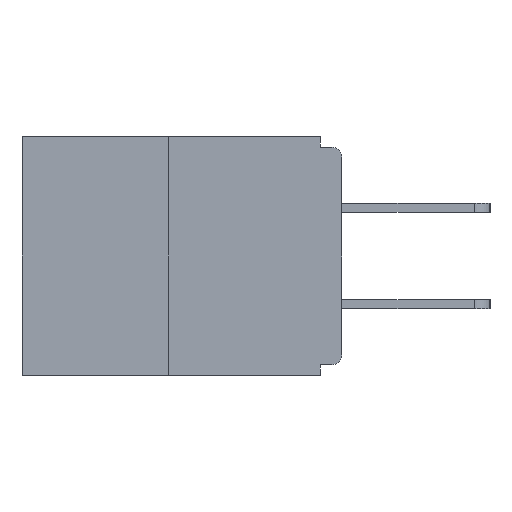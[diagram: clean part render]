
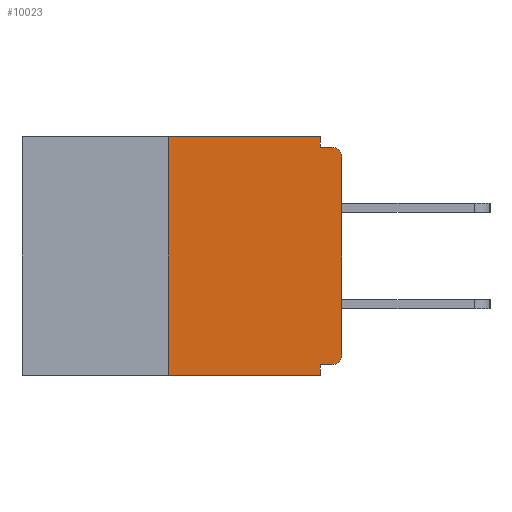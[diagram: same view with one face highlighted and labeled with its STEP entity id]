
A CAD part, left-side view. The second image highlights one B-rep face of the part: STEP entity #10023.
In plain terms, the highlighted planar face has unit normal (-1, 0, 0).
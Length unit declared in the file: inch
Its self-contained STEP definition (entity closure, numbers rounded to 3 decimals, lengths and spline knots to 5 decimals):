
#547 = CARTESIAN_POINT ( 'NONE',  ( 0., 0.25, 0. ) ) ;
#806 = EDGE_CURVE ( 'NONE', #11763, #2201, #15070, .T. ) ;
#1167 = DIRECTION ( 'NONE',  ( 0., -1., 0. ) ) ;
#1571 = VECTOR ( 'NONE', #18775, 39.37008 ) ;
#1791 = EDGE_CURVE ( 'NONE', #5650, #12004, #2619, .T. ) ;
#1837 = DIRECTION ( 'NONE',  ( 0., 0., 1. ) ) ;
#2201 = VERTEX_POINT ( 'NONE', #16176 ) ;
#2619 = LINE ( 'NONE', #13761, #1571 ) ;
#2719 = CARTESIAN_POINT ( 'NONE',  ( 0., 0.031, 0. ) ) ;
#2844 = EDGE_LOOP ( 'NONE', ( #19851, #19224, #20400, #4843, #5907, #3986, #19819, #8966, #21171, #15029 ) ) ;
#2863 = VECTOR ( 'NONE', #1167, 39.37008 ) ;
#2979 = DIRECTION ( 'NONE',  ( -1., 0., 0. ) ) ;
#3057 = VERTEX_POINT ( 'NONE', #15165 ) ;
#3121 = PLANE ( 'NONE',  #12375 ) ;
#3280 = VERTEX_POINT ( 'NONE', #2719 ) ;
#3747 = VERTEX_POINT ( 'NONE', #6689 ) ;
#3932 = VERTEX_POINT ( 'NONE', #12876 ) ;
#3986 = ORIENTED_EDGE ( 'NONE', *, *, #5070, .T. ) ;
#4358 = EDGE_CURVE ( 'NONE', #3280, #3932, #9480, .T. ) ;
#4368 = CARTESIAN_POINT ( 'NONE',  ( 0., 0., -0.313 ) ) ;
#4381 = DIRECTION ( 'NONE',  ( 0., 1., 0. ) ) ;
#4698 = DIRECTION ( 'NONE',  ( 0., 0., -1. ) ) ;
#4843 = ORIENTED_EDGE ( 'NONE', *, *, #806, .F. ) ;
#4936 = CARTESIAN_POINT ( 'NONE',  ( 0., 0.46, 0. ) ) ;
#5070 = EDGE_CURVE ( 'NONE', #8528, #5650, #17501, .T. ) ;
#5142 = DIRECTION ( 'NONE',  ( -1., 0., 0. ) ) ;
#5148 = CARTESIAN_POINT ( 'NONE',  ( 0., 0.25, 0. ) ) ;
#5252 = CARTESIAN_POINT ( 'NONE',  ( 0., 0.031, -0.343 ) ) ;
#5650 = VERTEX_POINT ( 'NONE', #4368 ) ;
#5907 = ORIENTED_EDGE ( 'NONE', *, *, #20218, .F. ) ;
#6101 = CARTESIAN_POINT ( 'NONE',  ( 0., 0., -0.015 ) ) ;
#6421 = LINE ( 'NONE', #4936, #18663 ) ;
#6689 = CARTESIAN_POINT ( 'NONE',  ( 0., 0.25, -0.343 ) ) ;
#7556 = VECTOR ( 'NONE', #4381, 39.37008 ) ;
#7719 = DIRECTION ( 'NONE',  ( 0., -1., 0. ) ) ;
#7765 = EDGE_CURVE ( 'NONE', #3932, #3057, #11703, .T. ) ;
#7767 = EDGE_CURVE ( 'NONE', #3747, #2201, #15612, .T. ) ;
#8050 = CARTESIAN_POINT ( 'NONE',  ( 0., 0.46, 0. ) ) ;
#8097 = CARTESIAN_POINT ( 'NONE',  ( 0., 0., -0.03 ) ) ;
#8465 = VECTOR ( 'NONE', #14899, 39.37008 ) ;
#8528 = VERTEX_POINT ( 'NONE', #13852 ) ;
#8966 = ORIENTED_EDGE ( 'NONE', *, *, #17107, .T. ) ;
#9126 = LINE ( 'NONE', #11038, #7556 ) ;
#9328 = EDGE_CURVE ( 'NONE', #3747, #17406, #17929, .T. ) ;
#9480 = LINE ( 'NONE', #13142, #8465 ) ;
#10023 = ADVANCED_FACE ( 'NONE', ( #17622 ), #3121, .F. ) ;
#11038 = CARTESIAN_POINT ( 'NONE',  ( 0., 0., -0.328 ) ) ;
#11395 = EDGE_CURVE ( 'NONE', #17406, #3280, #6421, .T. ) ;
#11703 = LINE ( 'NONE', #6101, #2863 ) ;
#11763 = VERTEX_POINT ( 'NONE', #19860 ) ;
#12004 = VERTEX_POINT ( 'NONE', #8097 ) ;
#12206 = AXIS2_PLACEMENT_3D ( 'NONE', #12943, #2979, #4698 ) ;
#12375 = AXIS2_PLACEMENT_3D ( 'NONE', #8050, #14751, #12997 ) ;
#12595 = AXIS2_PLACEMENT_3D ( 'NONE', #21159, #5142, #15428 ) ;
#12876 = CARTESIAN_POINT ( 'NONE',  ( 0., 0.031, -0.015 ) ) ;
#12943 = CARTESIAN_POINT ( 'NONE',  ( 0., 0.015, -0.03 ) ) ;
#12997 = DIRECTION ( 'NONE',  ( 0., 0., -1. ) ) ;
#13142 = CARTESIAN_POINT ( 'NONE',  ( 0., 0.031, 0. ) ) ;
#13761 = CARTESIAN_POINT ( 'NONE',  ( 0., 0., 0. ) ) ;
#13852 = CARTESIAN_POINT ( 'NONE',  ( 0., 0.015, -0.328 ) ) ;
#14751 = DIRECTION ( 'NONE',  ( 1., 0., 0. ) ) ;
#14802 = VECTOR ( 'NONE', #18476, 39.37008 ) ;
#14899 = DIRECTION ( 'NONE',  ( 0., 0., -1. ) ) ;
#15029 = ORIENTED_EDGE ( 'NONE', *, *, #4358, .F. ) ;
#15070 = LINE ( 'NONE', #5252, #14802 ) ;
#15165 = CARTESIAN_POINT ( 'NONE',  ( 0., 0.015, -0.015 ) ) ;
#15428 = DIRECTION ( 'NONE',  ( 0., 0., -1. ) ) ;
#15612 = LINE ( 'NONE', #16262, #17674 ) ;
#16176 = CARTESIAN_POINT ( 'NONE',  ( 0., 0.031, -0.343 ) ) ;
#16262 = CARTESIAN_POINT ( 'NONE',  ( 0., 0.46, -0.343 ) ) ;
#17107 = EDGE_CURVE ( 'NONE', #12004, #3057, #21233, .T. ) ;
#17406 = VERTEX_POINT ( 'NONE', #547 ) ;
#17501 = CIRCLE ( 'NONE', #12595, 0.015 ) ;
#17622 = FACE_OUTER_BOUND ( 'NONE', #2844, .T. ) ;
#17674 = VECTOR ( 'NONE', #7719, 39.37008 ) ;
#17929 = LINE ( 'NONE', #5148, #20034 ) ;
#18476 = DIRECTION ( 'NONE',  ( 0., 0., -1. ) ) ;
#18663 = VECTOR ( 'NONE', #21525, 39.37008 ) ;
#18775 = DIRECTION ( 'NONE',  ( 0., 0., 1. ) ) ;
#19224 = ORIENTED_EDGE ( 'NONE', *, *, #9328, .F. ) ;
#19819 = ORIENTED_EDGE ( 'NONE', *, *, #1791, .T. ) ;
#19851 = ORIENTED_EDGE ( 'NONE', *, *, #11395, .F. ) ;
#19860 = CARTESIAN_POINT ( 'NONE',  ( 0., 0.031, -0.328 ) ) ;
#20034 = VECTOR ( 'NONE', #1837, 39.37008 ) ;
#20218 = EDGE_CURVE ( 'NONE', #8528, #11763, #9126, .T. ) ;
#20400 = ORIENTED_EDGE ( 'NONE', *, *, #7767, .T. ) ;
#21159 = CARTESIAN_POINT ( 'NONE',  ( 0., 0.015, -0.313 ) ) ;
#21171 = ORIENTED_EDGE ( 'NONE', *, *, #7765, .F. ) ;
#21233 = CIRCLE ( 'NONE', #12206, 0.015 ) ;
#21525 = DIRECTION ( 'NONE',  ( 0., -1., 0. ) ) ;
